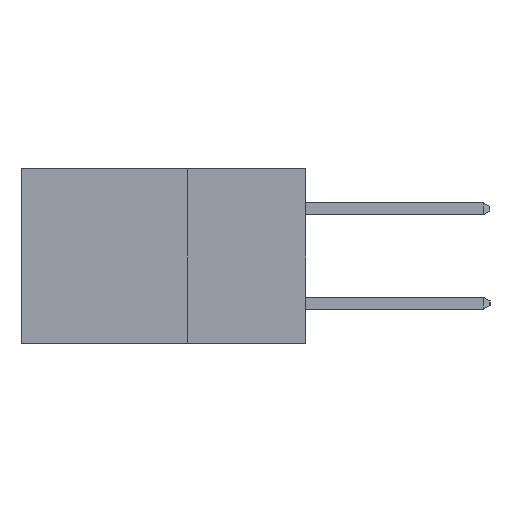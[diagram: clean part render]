
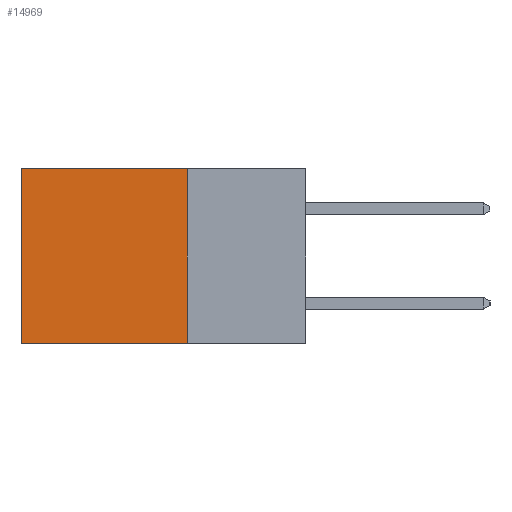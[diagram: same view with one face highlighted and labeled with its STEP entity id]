
A CAD part, left-side view. The second image highlights one B-rep face of the part: STEP entity #14969.
In plain terms, the highlighted planar face has unit normal (-1, 0, 0).
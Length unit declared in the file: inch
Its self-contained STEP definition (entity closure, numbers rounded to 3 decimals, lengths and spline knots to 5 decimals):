
#1450 = VERTEX_POINT ( 'NONE', #15269 ) ;
#1526 = VERTEX_POINT ( 'NONE', #7689 ) ;
#1860 = CARTESIAN_POINT ( 'NONE',  ( 0.2615, 0.25, -0.37 ) ) ;
#2456 = DIRECTION ( 'NONE',  ( 0., 1., 0. ) ) ;
#2564 = EDGE_CURVE ( 'NONE', #1526, #1450, #10168, .T. ) ;
#3406 = EDGE_CURVE ( 'NONE', #20355, #20654, #20482, .T. ) ;
#4046 = CARTESIAN_POINT ( 'NONE',  ( 0.2615, 0.6, -0.37 ) ) ;
#4098 = DIRECTION ( 'NONE',  ( 0., 0., -1. ) ) ;
#4717 = PLANE ( 'NONE',  #18218 ) ;
#4786 = CARTESIAN_POINT ( 'NONE',  ( 0.2615, 0.25, -0.37 ) ) ;
#5596 = EDGE_LOOP ( 'NONE', ( #6876, #19936, #13981, #13180 ) ) ;
#5802 = VECTOR ( 'NONE', #5864, 39.37008 ) ;
#5864 = DIRECTION ( 'NONE',  ( 0., 0., -1. ) ) ;
#6475 = DIRECTION ( 'NONE',  ( 0., 0., -1. ) ) ;
#6876 = ORIENTED_EDGE ( 'NONE', *, *, #3406, .T. ) ;
#7689 = CARTESIAN_POINT ( 'NONE',  ( 0.2615, 0.25, 0. ) ) ;
#10168 = LINE ( 'NONE', #1860, #5802 ) ;
#10320 = CARTESIAN_POINT ( 'NONE',  ( 0.2615, 0.6, -0.37 ) ) ;
#12496 = CARTESIAN_POINT ( 'NONE',  ( 0.2615, 0.25, -0.37 ) ) ;
#13180 = ORIENTED_EDGE ( 'NONE', *, *, #13284, .T. ) ;
#13284 = EDGE_CURVE ( 'NONE', #1526, #20355, #19719, .T. ) ;
#13981 = ORIENTED_EDGE ( 'NONE', *, *, #2564, .F. ) ;
#14969 = ADVANCED_FACE ( 'NONE', ( #16290 ), #4717, .F. ) ;
#15269 = CARTESIAN_POINT ( 'NONE',  ( 0.2615, 0.25, -0.37 ) ) ;
#15359 = VECTOR ( 'NONE', #20235, 39.37008 ) ;
#16080 = VECTOR ( 'NONE', #4098, 39.37008 ) ;
#16290 = FACE_OUTER_BOUND ( 'NONE', #5596, .T. ) ;
#16359 = DIRECTION ( 'NONE',  ( 1., 0., 0. ) ) ;
#17163 = LINE ( 'NONE', #12496, #21040 ) ;
#17888 = EDGE_CURVE ( 'NONE', #1450, #20654, #17163, .T. ) ;
#18165 = CARTESIAN_POINT ( 'NONE',  ( 0.2615, 0.6, 0. ) ) ;
#18218 = AXIS2_PLACEMENT_3D ( 'NONE', #4786, #16359, #6475 ) ;
#18565 = CARTESIAN_POINT ( 'NONE',  ( 0.2615, 0.25, 0. ) ) ;
#19719 = LINE ( 'NONE', #18565, #15359 ) ;
#19936 = ORIENTED_EDGE ( 'NONE', *, *, #17888, .F. ) ;
#20235 = DIRECTION ( 'NONE',  ( 0., 1., 0. ) ) ;
#20355 = VERTEX_POINT ( 'NONE', #18165 ) ;
#20482 = LINE ( 'NONE', #10320, #16080 ) ;
#20654 = VERTEX_POINT ( 'NONE', #4046 ) ;
#21040 = VECTOR ( 'NONE', #2456, 39.37008 ) ;
